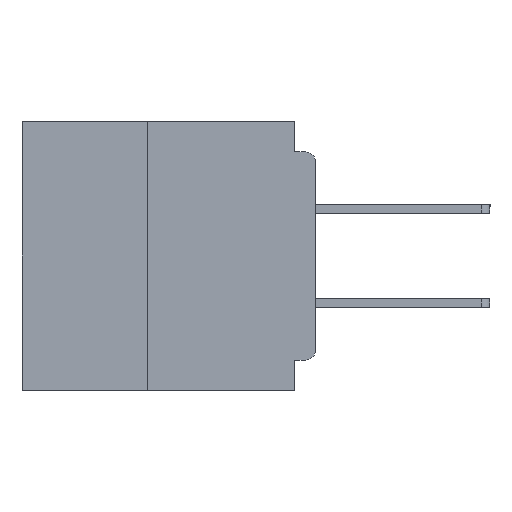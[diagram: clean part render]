
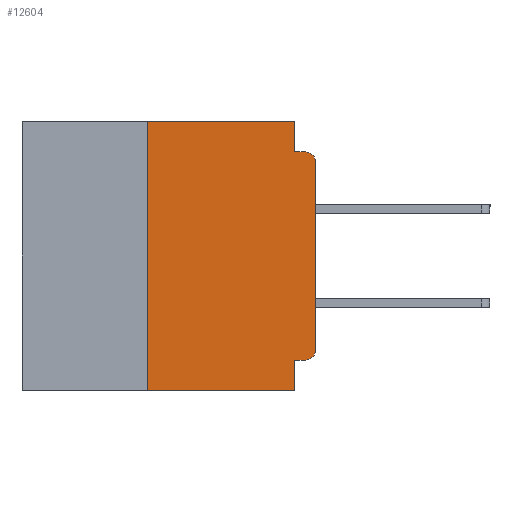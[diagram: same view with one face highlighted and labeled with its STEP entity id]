
A CAD part, left-side view. The second image highlights one B-rep face of the part: STEP entity #12604.
In plain terms, the highlighted planar face has unit normal (-1, 0, 0).
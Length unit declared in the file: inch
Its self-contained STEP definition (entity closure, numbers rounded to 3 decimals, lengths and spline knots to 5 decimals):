
#37 = LINE ( 'NONE', #39374, #11993 ) ;
#108 = DIRECTION ( 'NONE',  ( 0., -1., 0. ) ) ;
#1323 = VECTOR ( 'NONE', #2554, 39.37008 ) ;
#2045 = LINE ( 'NONE', #8004, #11457 ) ;
#2554 = DIRECTION ( 'NONE',  ( 0., -1., 0. ) ) ;
#3827 = VERTEX_POINT ( 'NONE', #50052 ) ;
#4664 = EDGE_CURVE ( 'NONE', #28593, #11227, #37, .T. ) ;
#4718 = DIRECTION ( 'NONE',  ( 0., 0., -1. ) ) ;
#4896 = VECTOR ( 'NONE', #49516, 39.37008 ) ;
#5262 = VECTOR ( 'NONE', #7291, 39.37008 ) ;
#5941 = EDGE_CURVE ( 'NONE', #10933, #26080, #40810, .T. ) ;
#6220 = ORIENTED_EDGE ( 'NONE', *, *, #10802, .T. ) ;
#6869 = CARTESIAN_POINT ( 'NONE',  ( 0., 0., -0.355 ) ) ;
#7042 = DIRECTION ( 'NONE',  ( 0., 1., 0. ) ) ;
#7291 = DIRECTION ( 'NONE',  ( 0., 0., -1. ) ) ;
#8004 = CARTESIAN_POINT ( 'NONE',  ( 0., 0., -0.045 ) ) ;
#10044 = EDGE_CURVE ( 'NONE', #36446, #41226, #2045, .T. ) ;
#10802 = EDGE_CURVE ( 'NONE', #28593, #48927, #13289, .T. ) ;
#10870 = VERTEX_POINT ( 'NONE', #35209 ) ;
#10933 = VERTEX_POINT ( 'NONE', #27561 ) ;
#11227 = VERTEX_POINT ( 'NONE', #29287 ) ;
#11276 = DIRECTION ( 'NONE',  ( 0., 0., 1. ) ) ;
#11294 = ORIENTED_EDGE ( 'NONE', *, *, #5941, .F. ) ;
#11457 = VECTOR ( 'NONE', #108, 39.37008 ) ;
#11993 = VECTOR ( 'NONE', #11276, 39.37008 ) ;
#12506 = LINE ( 'NONE', #12556, #23245 ) ;
#12556 = CARTESIAN_POINT ( 'NONE',  ( 0., 0., 0. ) ) ;
#12604 = ADVANCED_FACE ( 'NONE', ( #26365 ), #50551, .F. ) ;
#13289 = LINE ( 'NONE', #34696, #1323 ) ;
#14711 = DIRECTION ( 'NONE',  ( 0., 0., -1. ) ) ;
#14791 = CARTESIAN_POINT ( 'NONE',  ( 0., 0.015, -0.045 ) ) ;
#15097 = DIRECTION ( 'NONE',  ( -1., 0., 0. ) ) ;
#16608 = VECTOR ( 'NONE', #4718, 39.37008 ) ;
#16652 = DIRECTION ( 'NONE',  ( 0., 0., 1. ) ) ;
#17267 = LINE ( 'NONE', #27413, #5262 ) ;
#17785 = ORIENTED_EDGE ( 'NONE', *, *, #25880, .T. ) ;
#18085 = EDGE_CURVE ( 'NONE', #11227, #36287, #47556, .T. ) ;
#18877 = ORIENTED_EDGE ( 'NONE', *, *, #10044, .F. ) ;
#20665 = EDGE_CURVE ( 'NONE', #26080, #48927, #48495, .T. ) ;
#20944 = EDGE_CURVE ( 'NONE', #3827, #41226, #46622, .T. ) ;
#22646 = CARTESIAN_POINT ( 'NONE',  ( 0., 0.437, 0. ) ) ;
#23245 = VECTOR ( 'NONE', #16652, 39.37008 ) ;
#23455 = AXIS2_PLACEMENT_3D ( 'NONE', #39100, #15097, #43096 ) ;
#24080 = DIRECTION ( 'NONE',  ( -1., 0., 0. ) ) ;
#24203 = CARTESIAN_POINT ( 'NONE',  ( 0., 0.25, -0.4 ) ) ;
#25654 = DIRECTION ( 'NONE',  ( 0., 0., -1. ) ) ;
#25880 = EDGE_CURVE ( 'NONE', #10933, #10870, #44454, .T. ) ;
#26080 = VERTEX_POINT ( 'NONE', #41911 ) ;
#26365 = FACE_OUTER_BOUND ( 'NONE', #41242, .T. ) ;
#27413 = CARTESIAN_POINT ( 'NONE',  ( 0., 0.031, 0. ) ) ;
#27561 = CARTESIAN_POINT ( 'NONE',  ( 0., 0.015, -0.355 ) ) ;
#28491 = EDGE_CURVE ( 'NONE', #36287, #36446, #17267, .T. ) ;
#28593 = VERTEX_POINT ( 'NONE', #24203 ) ;
#28828 = ORIENTED_EDGE ( 'NONE', *, *, #36516, .T. ) ;
#29287 = CARTESIAN_POINT ( 'NONE',  ( 0., 0.25, 0. ) ) ;
#30225 = VECTOR ( 'NONE', #7042, 39.37008 ) ;
#30974 = ORIENTED_EDGE ( 'NONE', *, *, #28491, .F. ) ;
#32277 = CARTESIAN_POINT ( 'NONE',  ( 0., 0.031, -0.045 ) ) ;
#34477 = ORIENTED_EDGE ( 'NONE', *, *, #18085, .F. ) ;
#34696 = CARTESIAN_POINT ( 'NONE',  ( 0., 0.437, -0.4 ) ) ;
#35046 = AXIS2_PLACEMENT_3D ( 'NONE', #47994, #24080, #25654 ) ;
#35209 = CARTESIAN_POINT ( 'NONE',  ( 0., 0., -0.34 ) ) ;
#36287 = VERTEX_POINT ( 'NONE', #43090 ) ;
#36446 = VERTEX_POINT ( 'NONE', #32277 ) ;
#36516 = EDGE_CURVE ( 'NONE', #10870, #3827, #12506, .T. ) ;
#38736 = DIRECTION ( 'NONE',  ( 1., 0., 0. ) ) ;
#39100 = CARTESIAN_POINT ( 'NONE',  ( 0., 0.015, -0.06 ) ) ;
#39374 = CARTESIAN_POINT ( 'NONE',  ( 0., 0.25, -0.4 ) ) ;
#40810 = LINE ( 'NONE', #6869, #30225 ) ;
#41226 = VERTEX_POINT ( 'NONE', #14791 ) ;
#41242 = EDGE_LOOP ( 'NONE', ( #28828, #44426, #18877, #30974, #34477, #46703, #6220, #43564, #11294, #17785 ) ) ;
#41911 = CARTESIAN_POINT ( 'NONE',  ( 0., 0.031, -0.355 ) ) ;
#43090 = CARTESIAN_POINT ( 'NONE',  ( 0., 0.031, 0. ) ) ;
#43096 = DIRECTION ( 'NONE',  ( 0., 0., -1. ) ) ;
#43564 = ORIENTED_EDGE ( 'NONE', *, *, #20665, .F. ) ;
#44426 = ORIENTED_EDGE ( 'NONE', *, *, #20944, .T. ) ;
#44454 = CIRCLE ( 'NONE', #35046, 0.015 ) ;
#45060 = CARTESIAN_POINT ( 'NONE',  ( 0., 0.031, -0.4 ) ) ;
#45316 = CARTESIAN_POINT ( 'NONE',  ( 0., 0.031, -0.4 ) ) ;
#45526 = CARTESIAN_POINT ( 'NONE',  ( 0., 0.437, 0. ) ) ;
#46622 = CIRCLE ( 'NONE', #23455, 0.015 ) ;
#46703 = ORIENTED_EDGE ( 'NONE', *, *, #4664, .F. ) ;
#47556 = LINE ( 'NONE', #45526, #4896 ) ;
#47994 = CARTESIAN_POINT ( 'NONE',  ( 0., 0.015, -0.34 ) ) ;
#48495 = LINE ( 'NONE', #45060, #16608 ) ;
#48927 = VERTEX_POINT ( 'NONE', #45316 ) ;
#49516 = DIRECTION ( 'NONE',  ( 0., -1., 0. ) ) ;
#50052 = CARTESIAN_POINT ( 'NONE',  ( 0., 0., -0.06 ) ) ;
#50551 = PLANE ( 'NONE',  #51263 ) ;
#51263 = AXIS2_PLACEMENT_3D ( 'NONE', #22646, #38736, #14711 ) ;
